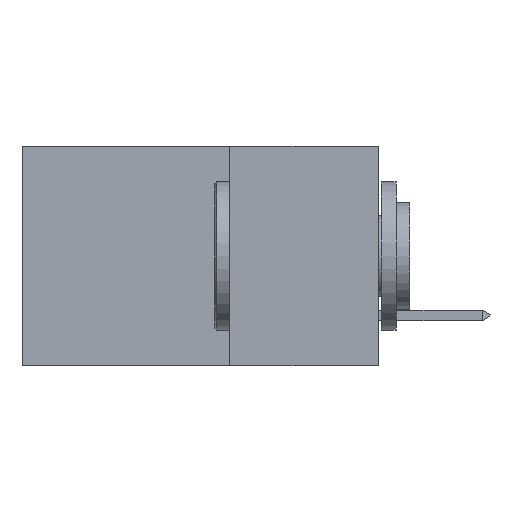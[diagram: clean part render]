
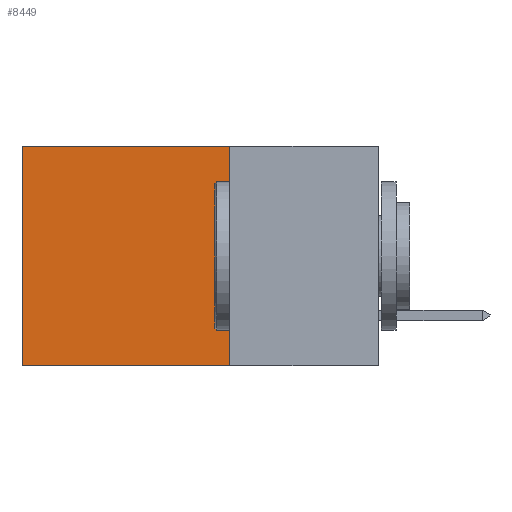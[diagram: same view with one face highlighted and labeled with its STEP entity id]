
A CAD part, left-side view. The second image highlights one B-rep face of the part: STEP entity #8449.
In plain terms, the highlighted planar face has unit normal (-1, 0, 0).
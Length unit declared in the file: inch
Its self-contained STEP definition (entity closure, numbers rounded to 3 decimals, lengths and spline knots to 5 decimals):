
#171 = VECTOR ( 'NONE', #873, 39.37008 ) ;
#240 = EDGE_CURVE ( 'NONE', #13510, #7992, #4618, .T. ) ;
#553 = ORIENTED_EDGE ( 'NONE', *, *, #240, .T. ) ;
#873 = DIRECTION ( 'NONE',  ( 0., 0., -1. ) ) ;
#939 = PLANE ( 'NONE',  #13938 ) ;
#1111 = EDGE_CURVE ( 'NONE', #13510, #8649, #3255, .T. ) ;
#1574 = CARTESIAN_POINT ( 'NONE',  ( 0.2615, 0.6, 0. ) ) ;
#1887 = DIRECTION ( 'NONE',  ( 1., 0., 0. ) ) ;
#2504 = ORIENTED_EDGE ( 'NONE', *, *, #10446, .F. ) ;
#2626 = CARTESIAN_POINT ( 'NONE',  ( 0.2615, 0.25, -0.37 ) ) ;
#3197 = ORIENTED_EDGE ( 'NONE', *, *, #1111, .F. ) ;
#3255 = LINE ( 'NONE', #12182, #171 ) ;
#3293 = CARTESIAN_POINT ( 'NONE',  ( 0.2615, 0.6, -0.37 ) ) ;
#3441 = ORIENTED_EDGE ( 'NONE', *, *, #11029, .T. ) ;
#3711 = LINE ( 'NONE', #2626, #9650 ) ;
#4377 = LINE ( 'NONE', #3293, #9892 ) ;
#4618 = LINE ( 'NONE', #5855, #13982 ) ;
#5855 = CARTESIAN_POINT ( 'NONE',  ( 0.2615, 0.25, 0. ) ) ;
#5989 = EDGE_LOOP ( 'NONE', ( #3441, #2504, #3197, #553 ) ) ;
#7099 = CARTESIAN_POINT ( 'NONE',  ( 0.2615, 0.25, 0. ) ) ;
#7992 = VERTEX_POINT ( 'NONE', #1574 ) ;
#8449 = ADVANCED_FACE ( 'NONE', ( #10271 ), #939, .F. ) ;
#8614 = CARTESIAN_POINT ( 'NONE',  ( 0.2615, 0.25, -0.37 ) ) ;
#8649 = VERTEX_POINT ( 'NONE', #8614 ) ;
#9355 = VERTEX_POINT ( 'NONE', #14145 ) ;
#9650 = VECTOR ( 'NONE', #11526, 39.37008 ) ;
#9892 = VECTOR ( 'NONE', #12208, 39.37008 ) ;
#10161 = DIRECTION ( 'NONE',  ( 0., 1., 0. ) ) ;
#10271 = FACE_OUTER_BOUND ( 'NONE', #5989, .T. ) ;
#10446 = EDGE_CURVE ( 'NONE', #8649, #9355, #3711, .T. ) ;
#10642 = DIRECTION ( 'NONE',  ( 0., 0., -1. ) ) ;
#11029 = EDGE_CURVE ( 'NONE', #7992, #9355, #4377, .T. ) ;
#11526 = DIRECTION ( 'NONE',  ( 0., 1., 0. ) ) ;
#11821 = CARTESIAN_POINT ( 'NONE',  ( 0.2615, 0.25, -0.37 ) ) ;
#12182 = CARTESIAN_POINT ( 'NONE',  ( 0.2615, 0.25, -0.37 ) ) ;
#12208 = DIRECTION ( 'NONE',  ( 0., 0., -1. ) ) ;
#13510 = VERTEX_POINT ( 'NONE', #7099 ) ;
#13938 = AXIS2_PLACEMENT_3D ( 'NONE', #11821, #1887, #10642 ) ;
#13982 = VECTOR ( 'NONE', #10161, 39.37008 ) ;
#14145 = CARTESIAN_POINT ( 'NONE',  ( 0.2615, 0.6, -0.37 ) ) ;
